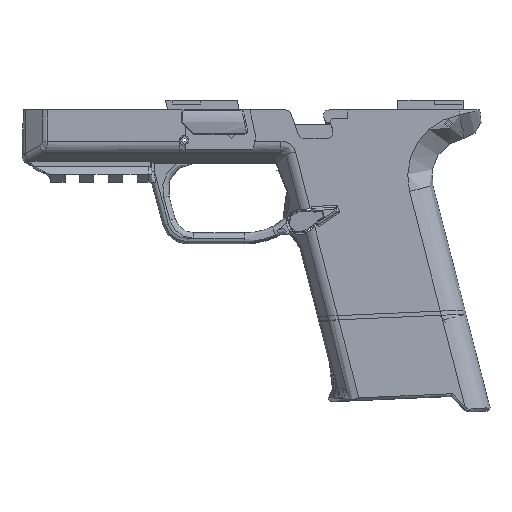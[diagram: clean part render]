
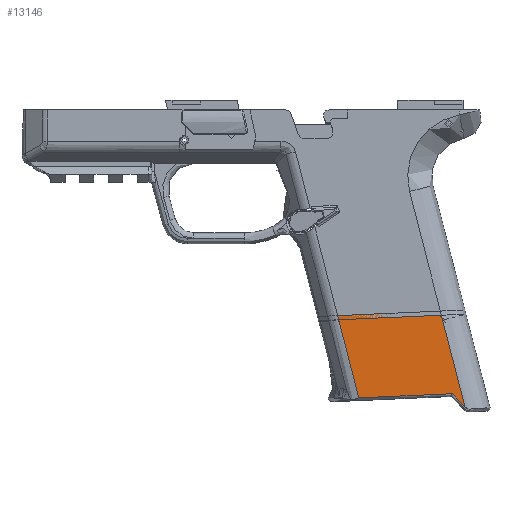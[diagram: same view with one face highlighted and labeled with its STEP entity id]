
A CAD part, left-side view. The second image highlights one B-rep face of the part: STEP entity #13146.
In plain terms, the highlighted face is planar.
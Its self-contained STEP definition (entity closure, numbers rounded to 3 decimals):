
#1066=PLANE('',#14392);
#1757=FACE_OUTER_BOUND('',#2512,.T.);
#2512=EDGE_LOOP('',(#11897,#11898,#11899,#11900,#11901));
#3570=LINE('',#25109,#4711);
#3590=LINE('',#25955,#4731);
#3604=LINE('',#26376,#4745);
#3605=LINE('',#26380,#4746);
#3606=LINE('',#26381,#4747);
#4711=VECTOR('',#17481,10.);
#4731=VECTOR('',#17573,10.);
#4745=VECTOR('',#17645,10.);
#4746=VECTOR('',#17650,10.);
#4747=VECTOR('',#17651,10.);
#6263=VERTEX_POINT('',#25087);
#6265=VERTEX_POINT('',#25107);
#6319=VERTEX_POINT('',#25954);
#6338=VERTEX_POINT('',#26217);
#6346=VERTEX_POINT('',#26379);
#8095=EDGE_CURVE('',#6265,#6263,#3570,.T.);
#8177=EDGE_CURVE('',#6319,#6263,#3590,.T.);
#8222=EDGE_CURVE('',#6338,#6265,#3604,.T.);
#8223=EDGE_CURVE('',#6346,#6338,#3605,.T.);
#8224=EDGE_CURVE('',#6346,#6319,#3606,.T.);
#11897=ORIENTED_EDGE('',*,*,#8095,.F.);
#11898=ORIENTED_EDGE('',*,*,#8222,.F.);
#11899=ORIENTED_EDGE('',*,*,#8223,.F.);
#11900=ORIENTED_EDGE('',*,*,#8224,.T.);
#11901=ORIENTED_EDGE('',*,*,#8177,.T.);
#13146=ADVANCED_FACE('',(#1757),#1066,.T.);
#14392=AXIS2_PLACEMENT_3D('',#26378,#17648,#17649);
#17481=DIRECTION('',(0.,0.999,0.044));
#17573=DIRECTION('',(0.,-0.249,0.969));
#17645=DIRECTION('',(0.,0.697,-0.717));
#17648=DIRECTION('center_axis',(1.,0.,0.));
#17649=DIRECTION('ref_axis',(0.,0.999,0.044));
#17650=DIRECTION('',(0.,-0.249,0.969));
#17651=DIRECTION('',(0.,0.999,0.044));
#25087=CARTESIAN_POINT('',(22.175,-44.727,96.906));
#25107=CARTESIAN_POINT('',(22.175,-78.67,95.402));
#25109=CARTESIAN_POINT('',(22.175,-44.598,96.911));
#25954=CARTESIAN_POINT('',(22.175,-37.062,67.087));
#25955=CARTESIAN_POINT('',(22.175,-37.062,67.087));
#26217=CARTESIAN_POINT('',(22.175,-83.249,100.107));
#26376=CARTESIAN_POINT('',(22.175,-73.025,89.603));
#26378=CARTESIAN_POINT('Origin',(22.175,-74.337,65.435));
#26379=CARTESIAN_POINT('',(22.175,-74.337,65.435));
#26380=CARTESIAN_POINT('',(22.175,-74.337,65.435));
#26381=CARTESIAN_POINT('',(22.175,-40.4,66.939));
